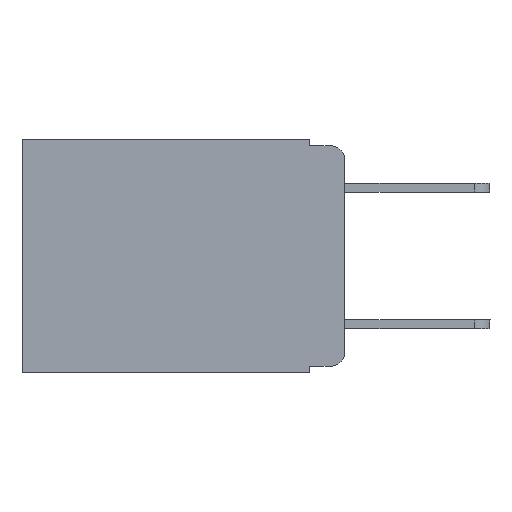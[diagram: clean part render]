
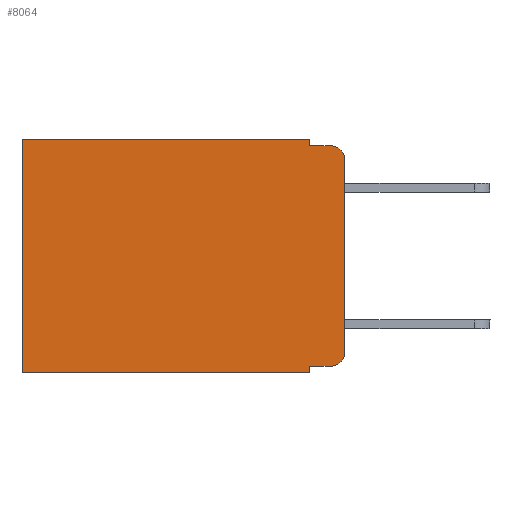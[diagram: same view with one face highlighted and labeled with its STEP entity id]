
A CAD part, left-side view. The second image highlights one B-rep face of the part: STEP entity #8064.
In plain terms, the highlighted planar face has unit normal (-1, 0, 0).
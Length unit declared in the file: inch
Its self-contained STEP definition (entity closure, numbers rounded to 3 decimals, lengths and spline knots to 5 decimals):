
#62 = ORIENTED_EDGE ( 'NONE', *, *, #10235, .F. ) ;
#103 = EDGE_CURVE ( 'NONE', #195, #6900, #3786, .T. ) ;
#161 = VECTOR ( 'NONE', #1937, 39.37008 ) ;
#195 = VERTEX_POINT ( 'NONE', #8864 ) ;
#332 = CARTESIAN_POINT ( 'NONE',  ( 0.298, 0., 0. ) ) ;
#415 = CARTESIAN_POINT ( 'NONE',  ( 0.298, 0.02, -0.333 ) ) ;
#416 = EDGE_CURVE ( 'NONE', #4793, #2527, #3486, .T. ) ;
#458 = CARTESIAN_POINT ( 'NONE',  ( 0.298, 0.051, -0.333 ) ) ;
#592 = LINE ( 'NONE', #8275, #971 ) ;
#653 = VECTOR ( 'NONE', #7178, 39.37008 ) ;
#856 = LINE ( 'NONE', #9242, #4068 ) ;
#971 = VECTOR ( 'NONE', #9077, 39.37008 ) ;
#1120 = DIRECTION ( 'NONE',  ( 0., 0., -1. ) ) ;
#1199 = VERTEX_POINT ( 'NONE', #5546 ) ;
#1271 = LINE ( 'NONE', #9896, #2361 ) ;
#1285 = CARTESIAN_POINT ( 'NONE',  ( 0.298, 0., -0.313 ) ) ;
#1539 = AXIS2_PLACEMENT_3D ( 'NONE', #9644, #7377, #3882 ) ;
#1610 = VERTEX_POINT ( 'NONE', #3909 ) ;
#1862 = ORIENTED_EDGE ( 'NONE', *, *, #103, .T. ) ;
#1937 = DIRECTION ( 'NONE',  ( 0., -1., 0. ) ) ;
#1943 = VERTEX_POINT ( 'NONE', #3757 ) ;
#1977 = VERTEX_POINT ( 'NONE', #9371 ) ;
#2024 = ORIENTED_EDGE ( 'NONE', *, *, #2289, .F. ) ;
#2061 = LINE ( 'NONE', #9041, #6037 ) ;
#2289 = EDGE_CURVE ( 'NONE', #5755, #1199, #2741, .T. ) ;
#2361 = VECTOR ( 'NONE', #5273, 39.37008 ) ;
#2527 = VERTEX_POINT ( 'NONE', #1285 ) ;
#2651 = DIRECTION ( 'NONE',  ( 1., 0., 0. ) ) ;
#2689 = PLANE ( 'NONE',  #7490 ) ;
#2741 = LINE ( 'NONE', #6897, #8536 ) ;
#2881 = LINE ( 'NONE', #9528, #653 ) ;
#2994 = CARTESIAN_POINT ( 'NONE',  ( 0.298, 0.051, -0.333 ) ) ;
#3486 = CIRCLE ( 'NONE', #1539, 0.02 ) ;
#3513 = ORIENTED_EDGE ( 'NONE', *, *, #6182, .F. ) ;
#3757 = CARTESIAN_POINT ( 'NONE',  ( 0.298, 0.051, 0. ) ) ;
#3786 = CIRCLE ( 'NONE', #7000, 0.02 ) ;
#3882 = DIRECTION ( 'NONE',  ( 0., 0., -1. ) ) ;
#3909 = CARTESIAN_POINT ( 'NONE',  ( 0.298, 0.473, 0. ) ) ;
#3917 = ORIENTED_EDGE ( 'NONE', *, *, #7191, .T. ) ;
#4068 = VECTOR ( 'NONE', #5328, 39.37008 ) ;
#4325 = ORIENTED_EDGE ( 'NONE', *, *, #9389, .F. ) ;
#4374 = LINE ( 'NONE', #458, #161 ) ;
#4781 = VERTEX_POINT ( 'NONE', #8382 ) ;
#4793 = VERTEX_POINT ( 'NONE', #415 ) ;
#5201 = FACE_OUTER_BOUND ( 'NONE', #8744, .T. ) ;
#5273 = DIRECTION ( 'NONE',  ( 0., 1., 0. ) ) ;
#5286 = DIRECTION ( 'NONE',  ( 0., 0., -1. ) ) ;
#5328 = DIRECTION ( 'NONE',  ( 0., 0., -1. ) ) ;
#5381 = DIRECTION ( 'NONE',  ( 0., 1., 0. ) ) ;
#5546 = CARTESIAN_POINT ( 'NONE',  ( 0.298, 0.051, -0.343 ) ) ;
#5618 = ORIENTED_EDGE ( 'NONE', *, *, #416, .T. ) ;
#5663 = EDGE_CURVE ( 'NONE', #5755, #4793, #4374, .T. ) ;
#5728 = CARTESIAN_POINT ( 'NONE',  ( 0.298, 0.02, -0.01 ) ) ;
#5755 = VERTEX_POINT ( 'NONE', #2994 ) ;
#5823 = DIRECTION ( 'NONE',  ( 0., 0., -1. ) ) ;
#5930 = ORIENTED_EDGE ( 'NONE', *, *, #9312, .T. ) ;
#6037 = VECTOR ( 'NONE', #5823, 39.37008 ) ;
#6113 = DIRECTION ( 'NONE',  ( 0., 0., -1. ) ) ;
#6182 = EDGE_CURVE ( 'NONE', #4781, #6900, #2881, .T. ) ;
#6648 = VECTOR ( 'NONE', #5381, 39.37008 ) ;
#6897 = CARTESIAN_POINT ( 'NONE',  ( 0.298, 0.051, 0. ) ) ;
#6900 = VERTEX_POINT ( 'NONE', #5728 ) ;
#6958 = DIRECTION ( 'NONE',  ( -1., 0., 0. ) ) ;
#7000 = AXIS2_PLACEMENT_3D ( 'NONE', #8558, #6958, #6113 ) ;
#7178 = DIRECTION ( 'NONE',  ( 0., -1., 0. ) ) ;
#7191 = EDGE_CURVE ( 'NONE', #1943, #1610, #1271, .T. ) ;
#7377 = DIRECTION ( 'NONE',  ( -1., 0., 0. ) ) ;
#7490 = AXIS2_PLACEMENT_3D ( 'NONE', #332, #2651, #1120 ) ;
#7756 = ORIENTED_EDGE ( 'NONE', *, *, #8836, .F. ) ;
#8064 = ADVANCED_FACE ( 'NONE', ( #5201 ), #2689, .F. ) ;
#8275 = CARTESIAN_POINT ( 'NONE',  ( 0.298, 0., 0. ) ) ;
#8324 = CARTESIAN_POINT ( 'NONE',  ( 0.298, 0., -0.343 ) ) ;
#8382 = CARTESIAN_POINT ( 'NONE',  ( 0.298, 0.051, -0.01 ) ) ;
#8536 = VECTOR ( 'NONE', #5286, 39.37008 ) ;
#8558 = CARTESIAN_POINT ( 'NONE',  ( 0.298, 0.02, -0.03 ) ) ;
#8744 = EDGE_LOOP ( 'NONE', ( #4325, #1862, #3513, #62, #3917, #5930, #7756, #2024, #9452, #5618 ) ) ;
#8749 = LINE ( 'NONE', #8324, #6648 ) ;
#8836 = EDGE_CURVE ( 'NONE', #1199, #1977, #8749, .T. ) ;
#8864 = CARTESIAN_POINT ( 'NONE',  ( 0.298, 0., -0.03 ) ) ;
#9041 = CARTESIAN_POINT ( 'NONE',  ( 0.298, 0.473, 0. ) ) ;
#9077 = DIRECTION ( 'NONE',  ( 0., 0., -1. ) ) ;
#9242 = CARTESIAN_POINT ( 'NONE',  ( 0.298, 0.051, 0. ) ) ;
#9312 = EDGE_CURVE ( 'NONE', #1610, #1977, #2061, .T. ) ;
#9371 = CARTESIAN_POINT ( 'NONE',  ( 0.298, 0.473, -0.343 ) ) ;
#9389 = EDGE_CURVE ( 'NONE', #195, #2527, #592, .T. ) ;
#9452 = ORIENTED_EDGE ( 'NONE', *, *, #5663, .T. ) ;
#9528 = CARTESIAN_POINT ( 'NONE',  ( 0.298, 0.051, -0.01 ) ) ;
#9644 = CARTESIAN_POINT ( 'NONE',  ( 0.298, 0.02, -0.313 ) ) ;
#9896 = CARTESIAN_POINT ( 'NONE',  ( 0.298, 0., 0. ) ) ;
#10235 = EDGE_CURVE ( 'NONE', #1943, #4781, #856, .T. ) ;
